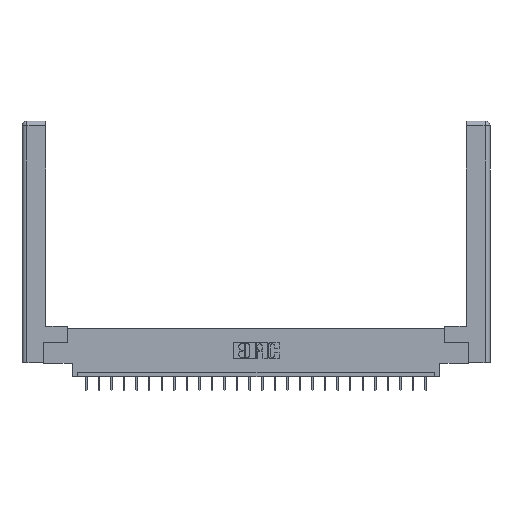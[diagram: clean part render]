
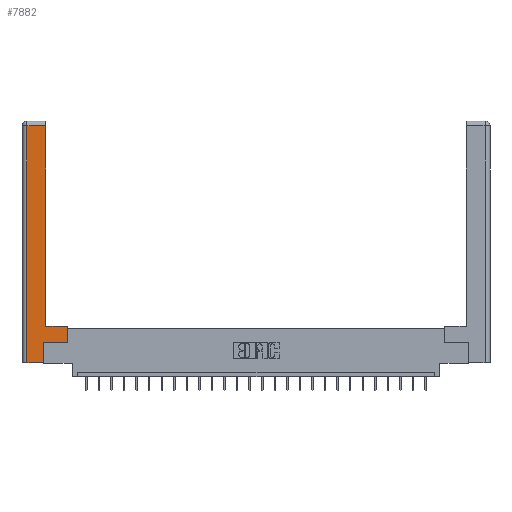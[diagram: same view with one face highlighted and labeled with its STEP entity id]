
A CAD part, top view. The second image highlights one B-rep face of the part: STEP entity #7882.
In plain terms, the highlighted planar face has unit normal (0, 0, 1).
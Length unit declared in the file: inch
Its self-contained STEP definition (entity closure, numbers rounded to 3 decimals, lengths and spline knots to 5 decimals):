
#548 = EDGE_CURVE ( 'NONE', #16156, #4802, #13460, .T. ) ;
#580 = EDGE_CURVE ( 'NONE', #21531, #5398, #6090, .T. ) ;
#1524 = VERTEX_POINT ( 'NONE', #8455 ) ;
#1893 = DIRECTION ( 'NONE',  ( 1., 0., 0. ) ) ;
#2188 = VECTOR ( 'NONE', #8517, 39.37008 ) ;
#2205 = VECTOR ( 'NONE', #7187, 39.37008 ) ;
#2260 = CARTESIAN_POINT ( 'NONE',  ( 0.0615, 2.94, 0. ) ) ;
#2378 = VECTOR ( 'NONE', #1893, 39.37008 ) ;
#2564 = CARTESIAN_POINT ( 'NONE',  ( 0.295, 0.45, 0. ) ) ;
#3436 = LINE ( 'NONE', #2564, #2188 ) ;
#3507 = VERTEX_POINT ( 'NONE', #8290 ) ;
#3598 = CARTESIAN_POINT ( 'NONE',  ( 0.265, 0., 0. ) ) ;
#3941 = VECTOR ( 'NONE', #9633, 39.37008 ) ;
#4066 = CARTESIAN_POINT ( 'NONE',  ( 0., 0., 0. ) ) ;
#4363 = ORIENTED_EDGE ( 'NONE', *, *, #548, .T. ) ;
#4747 = VECTOR ( 'NONE', #13878, 39.37008 ) ;
#4802 = VERTEX_POINT ( 'NONE', #3598 ) ;
#5367 = ORIENTED_EDGE ( 'NONE', *, *, #11706, .T. ) ;
#5386 = LINE ( 'NONE', #2260, #4747 ) ;
#5398 = VERTEX_POINT ( 'NONE', #8868 ) ;
#5604 = CARTESIAN_POINT ( 'NONE',  ( 0.565, 0.45, 0. ) ) ;
#6090 = LINE ( 'NONE', #5604, #3941 ) ;
#6129 = PLANE ( 'NONE',  #13988 ) ;
#6921 = LINE ( 'NONE', #21945, #16753 ) ;
#7158 = VECTOR ( 'NONE', #17880, 39.37008 ) ;
#7187 = DIRECTION ( 'NONE',  ( 1., 0., 0. ) ) ;
#7637 = EDGE_CURVE ( 'NONE', #4802, #7857, #6921, .T. ) ;
#7759 = DIRECTION ( 'NONE',  ( 0., 0., -1. ) ) ;
#7857 = VERTEX_POINT ( 'NONE', #9732 ) ;
#7882 = ADVANCED_FACE ( 'NONE', ( #24730 ), #6129, .F. ) ;
#8050 = ORIENTED_EDGE ( 'NONE', *, *, #14328, .T. ) ;
#8290 = CARTESIAN_POINT ( 'NONE',  ( 0.295, 2.94, 0. ) ) ;
#8455 = CARTESIAN_POINT ( 'NONE',  ( 0.0615, 2.94, 0. ) ) ;
#8517 = DIRECTION ( 'NONE',  ( -1., 0., 0. ) ) ;
#8868 = CARTESIAN_POINT ( 'NONE',  ( 0.565, 0.45, 0. ) ) ;
#8985 = LINE ( 'NONE', #19019, #2205 ) ;
#9633 = DIRECTION ( 'NONE',  ( 0., 1., 0. ) ) ;
#9732 = CARTESIAN_POINT ( 'NONE',  ( 0.265, 0.245, 0. ) ) ;
#9979 = EDGE_CURVE ( 'NONE', #3507, #1524, #5386, .T. ) ;
#10220 = DIRECTION ( 'NONE',  ( 0., 1., 0. ) ) ;
#10837 = LINE ( 'NONE', #15986, #7158 ) ;
#10880 = DIRECTION ( 'NONE',  ( 0., 1., 0. ) ) ;
#11175 = EDGE_CURVE ( 'NONE', #1524, #16156, #10837, .T. ) ;
#11333 = EDGE_CURVE ( 'NONE', #7857, #21531, #8985, .T. ) ;
#11706 = EDGE_CURVE ( 'NONE', #5398, #12716, #3436, .T. ) ;
#12293 = CARTESIAN_POINT ( 'NONE',  ( 0.565, 0.245, 0. ) ) ;
#12716 = VERTEX_POINT ( 'NONE', #21825 ) ;
#13460 = LINE ( 'NONE', #23478, #2378 ) ;
#13878 = DIRECTION ( 'NONE',  ( -1., 0., 0. ) ) ;
#13988 = AXIS2_PLACEMENT_3D ( 'NONE', #4066, #7759, #17721 ) ;
#14328 = EDGE_CURVE ( 'NONE', #12716, #3507, #16163, .T. ) ;
#15224 = ORIENTED_EDGE ( 'NONE', *, *, #9979, .T. ) ;
#15383 = ORIENTED_EDGE ( 'NONE', *, *, #580, .T. ) ;
#15758 = ORIENTED_EDGE ( 'NONE', *, *, #11333, .T. ) ;
#15986 = CARTESIAN_POINT ( 'NONE',  ( 0.0615, 0., 0. ) ) ;
#16003 = ORIENTED_EDGE ( 'NONE', *, *, #7637, .T. ) ;
#16156 = VERTEX_POINT ( 'NONE', #24014 ) ;
#16163 = LINE ( 'NONE', #18117, #23873 ) ;
#16753 = VECTOR ( 'NONE', #10220, 39.37008 ) ;
#17721 = DIRECTION ( 'NONE',  ( -1., 0., 0. ) ) ;
#17880 = DIRECTION ( 'NONE',  ( 0., -1., 0. ) ) ;
#18117 = CARTESIAN_POINT ( 'NONE',  ( 0.295, 3., 0. ) ) ;
#19019 = CARTESIAN_POINT ( 'NONE',  ( 0.565, 0.245, 0. ) ) ;
#19266 = EDGE_LOOP ( 'NONE', ( #8050, #15224, #24580, #4363, #16003, #15758, #15383, #5367 ) ) ;
#21531 = VERTEX_POINT ( 'NONE', #12293 ) ;
#21825 = CARTESIAN_POINT ( 'NONE',  ( 0.295, 0.45, 0. ) ) ;
#21945 = CARTESIAN_POINT ( 'NONE',  ( 0.265, 0.245, 0. ) ) ;
#23478 = CARTESIAN_POINT ( 'NONE',  ( 0.265, 0., 0. ) ) ;
#23873 = VECTOR ( 'NONE', #10880, 39.37008 ) ;
#24014 = CARTESIAN_POINT ( 'NONE',  ( 0.0615, 0., 0. ) ) ;
#24580 = ORIENTED_EDGE ( 'NONE', *, *, #11175, .T. ) ;
#24730 = FACE_OUTER_BOUND ( 'NONE', #19266, .T. ) ;
